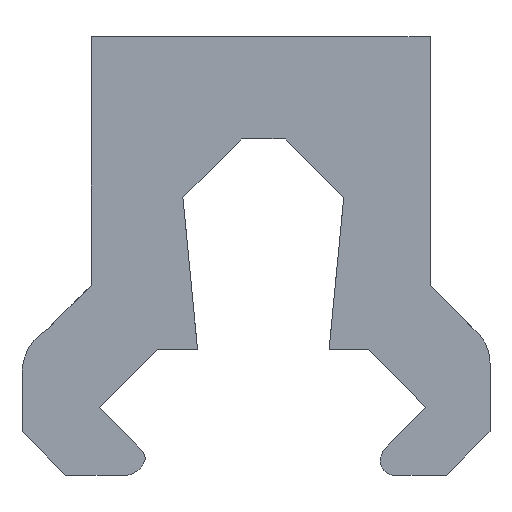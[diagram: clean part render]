
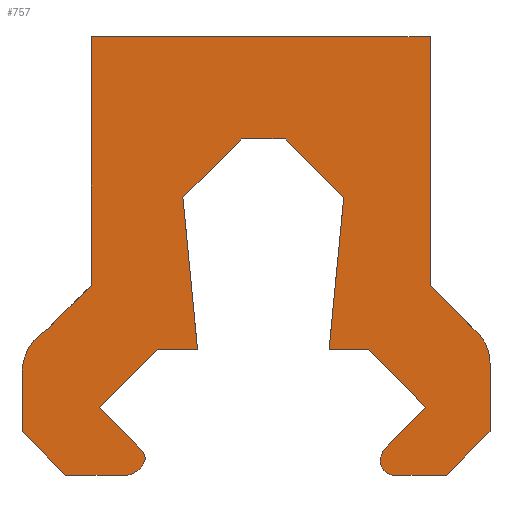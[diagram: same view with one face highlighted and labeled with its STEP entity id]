
A CAD part, left-side view. The second image highlights one B-rep face of the part: STEP entity #757.
In plain terms, the highlighted planar face has unit normal (-1, 0, 0).
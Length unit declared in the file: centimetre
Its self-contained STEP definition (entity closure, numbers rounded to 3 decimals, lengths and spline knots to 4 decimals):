
#36=LINE($,#1126,#114);
#41=LINE($,#1222,#119);
#46=LINE($,#1245,#124);
#49=LINE($,#1251,#127);
#50=LINE($,#1252,#128);
#51=LINE($,#1254,#129);
#52=LINE($,#1258,#130);
#53=LINE($,#1260,#131);
#54=LINE($,#1262,#132);
#55=LINE($,#1266,#133);
#56=LINE($,#1268,#134);
#57=LINE($,#1270,#135);
#58=LINE($,#1272,#136);
#59=LINE($,#1274,#137);
#60=LINE($,#1276,#138);
#61=LINE($,#1278,#139);
#62=LINE($,#1280,#140);
#63=LINE($,#1282,#141);
#64=LINE($,#1284,#142);
#65=LINE($,#1286,#143);
#66=LINE($,#1288,#144);
#67=LINE($,#1290,#145);
#68=LINE($,#1294,#146);
#69=LINE($,#1295,#147);
#114=VECTOR($,#853,1.7);
#119=VECTOR($,#878,0.4243);
#124=VECTOR($,#903,0.4678);
#127=VECTOR($,#908,1.7);
#128=VECTOR($,#909,2.3152);
#129=VECTOR($,#910,0.4243);
#130=VECTOR($,#913,0.397);
#131=VECTOR($,#914,0.4243);
#132=VECTOR($,#915,0.3982);
#133=VECTOR($,#918,0.0518);
#134=VECTOR($,#919,0.4193);
#135=VECTOR($,#920,0.5597);
#136=VECTOR($,#921,0.2742);
#137=VECTOR($,#922,1.0415);
#138=VECTOR($,#923,0.5657);
#139=VECTOR($,#924,0.3);
#140=VECTOR($,#925,0.5657);
#141=VECTOR($,#926,1.0415);
#142=VECTOR($,#927,0.2688);
#143=VECTOR($,#928,0.5597);
#144=VECTOR($,#929,0.4193);
#145=VECTOR($,#930,0.0346);
#146=VECTOR($,#933,0.35);
#147=VECTOR($,#934,0.4243);
#196=PLANE($,#810);
#231=CIRCLE($,#807,0.3);
#233=CIRCLE($,#811,0.35);
#234=CIRCLE($,#812,0.15);
#235=CIRCLE($,#813,0.1);
#253=FACE_OUTER_BOUND($,#297,.T.);
#297=EDGE_LOOP($,(#579,#580,#581,#582,#583,#584,#585,#586,#587,#588,#589,
#590,#591,#592,#593,#594,#595,#596,#597,#598,#599,#600,#601,#602,#603,#604,
#605,#606));
#343=VERTEX_POINT($,#1123);
#344=VERTEX_POINT($,#1125);
#356=VERTEX_POINT($,#1219);
#357=VERTEX_POINT($,#1221);
#363=VERTEX_POINT($,#1238);
#365=VERTEX_POINT($,#1244);
#367=VERTEX_POINT($,#1250);
#368=VERTEX_POINT($,#1253);
#369=VERTEX_POINT($,#1255);
#370=VERTEX_POINT($,#1257);
#371=VERTEX_POINT($,#1259);
#372=VERTEX_POINT($,#1261);
#373=VERTEX_POINT($,#1263);
#374=VERTEX_POINT($,#1265);
#375=VERTEX_POINT($,#1267);
#376=VERTEX_POINT($,#1269);
#377=VERTEX_POINT($,#1271);
#378=VERTEX_POINT($,#1273);
#379=VERTEX_POINT($,#1275);
#380=VERTEX_POINT($,#1277);
#381=VERTEX_POINT($,#1279);
#382=VERTEX_POINT($,#1281);
#383=VERTEX_POINT($,#1283);
#384=VERTEX_POINT($,#1285);
#385=VERTEX_POINT($,#1287);
#386=VERTEX_POINT($,#1289);
#387=VERTEX_POINT($,#1291);
#388=VERTEX_POINT($,#1293);
#422=EDGE_CURVE($,#344,#343,#36,.T.);
#438=EDGE_CURVE($,#357,#356,#41,.T.);
#445=EDGE_CURVE($,#357,#363,#231,.T.);
#448=EDGE_CURVE($,#363,#365,#46,.T.);
#451=EDGE_CURVE($,#356,#367,#49,.T.);
#452=EDGE_CURVE($,#344,#367,#50,.F.);
#453=EDGE_CURVE($,#343,#368,#51,.T.);
#454=EDGE_CURVE($,#369,#368,#233,.T.);
#455=EDGE_CURVE($,#370,#369,#52,.T.);
#456=EDGE_CURVE($,#371,#370,#53,.T.);
#457=EDGE_CURVE($,#372,#371,#54,.F.);
#458=EDGE_CURVE($,#373,#372,#234,.T.);
#459=EDGE_CURVE($,#374,#373,#55,.T.);
#460=EDGE_CURVE($,#375,#374,#56,.F.);
#461=EDGE_CURVE($,#376,#375,#57,.F.);
#462=EDGE_CURVE($,#377,#376,#58,.F.);
#463=EDGE_CURVE($,#377,#378,#59,.F.);
#464=EDGE_CURVE($,#379,#378,#60,.T.);
#465=EDGE_CURVE($,#379,#380,#61,.T.);
#466=EDGE_CURVE($,#381,#380,#62,.T.);
#467=EDGE_CURVE($,#381,#382,#63,.T.);
#468=EDGE_CURVE($,#383,#382,#64,.F.);
#469=EDGE_CURVE($,#384,#383,#65,.F.);
#470=EDGE_CURVE($,#385,#384,#66,.F.);
#471=EDGE_CURVE($,#386,#385,#67,.T.);
#472=EDGE_CURVE($,#387,#386,#235,.T.);
#473=EDGE_CURVE($,#388,#387,#68,.F.);
#474=EDGE_CURVE($,#365,#388,#69,.T.);
#579=ORIENTED_EDGE($,*,*,#445,.F.);
#580=ORIENTED_EDGE($,*,*,#438,.T.);
#581=ORIENTED_EDGE($,*,*,#451,.T.);
#582=ORIENTED_EDGE($,*,*,#452,.F.);
#583=ORIENTED_EDGE($,*,*,#422,.T.);
#584=ORIENTED_EDGE($,*,*,#453,.T.);
#585=ORIENTED_EDGE($,*,*,#454,.F.);
#586=ORIENTED_EDGE($,*,*,#455,.F.);
#587=ORIENTED_EDGE($,*,*,#456,.F.);
#588=ORIENTED_EDGE($,*,*,#457,.F.);
#589=ORIENTED_EDGE($,*,*,#458,.F.);
#590=ORIENTED_EDGE($,*,*,#459,.F.);
#591=ORIENTED_EDGE($,*,*,#460,.F.);
#592=ORIENTED_EDGE($,*,*,#461,.F.);
#593=ORIENTED_EDGE($,*,*,#462,.F.);
#594=ORIENTED_EDGE($,*,*,#463,.T.);
#595=ORIENTED_EDGE($,*,*,#464,.F.);
#596=ORIENTED_EDGE($,*,*,#465,.T.);
#597=ORIENTED_EDGE($,*,*,#466,.F.);
#598=ORIENTED_EDGE($,*,*,#467,.T.);
#599=ORIENTED_EDGE($,*,*,#468,.F.);
#600=ORIENTED_EDGE($,*,*,#469,.F.);
#601=ORIENTED_EDGE($,*,*,#470,.F.);
#602=ORIENTED_EDGE($,*,*,#471,.F.);
#603=ORIENTED_EDGE($,*,*,#472,.F.);
#604=ORIENTED_EDGE($,*,*,#473,.F.);
#605=ORIENTED_EDGE($,*,*,#474,.F.);
#606=ORIENTED_EDGE($,*,*,#448,.F.);
#757=ADVANCED_FACE($,(#253),#196,.F.);
#807=AXIS2_PLACEMENT_3D($,#1239,#896,#897);
#810=AXIS2_PLACEMENT_3D($,#1249,#906,#907);
#811=AXIS2_PLACEMENT_3D($,#1256,#911,#912);
#812=AXIS2_PLACEMENT_3D($,#1264,#916,#917);
#813=AXIS2_PLACEMENT_3D($,#1292,#931,#932);
#853=DIRECTION($,(0.,0.,-1.));
#878=DIRECTION($,(0.,0.707,0.707));
#896=DIRECTION('center_axis',(1.,0.,0.));
#897=DIRECTION('ref_axis',(0.,-0.633,0.774));
#903=DIRECTION($,(0.,0.,-1.));
#906=DIRECTION('center_axis',(1.,0.,0.));
#907=DIRECTION('ref_axis',(0.,0.,-1.));
#908=DIRECTION($,(0.,0.,1.));
#909=DIRECTION($,(0.,1.,0.));
#910=DIRECTION($,(0.,0.707,-0.707));
#911=DIRECTION('center_axis',(1.,0.,0.));
#912=DIRECTION('ref_axis',(0.,0.501,0.866));
#913=DIRECTION($,(0.,0.,1.));
#914=DIRECTION($,(0.,0.707,0.707));
#915=DIRECTION($,(0.,-1.,0.));
#916=DIRECTION('center_axis',(1.,0.,0.));
#917=DIRECTION('ref_axis',(0.,-0.976,-0.218));
#918=DIRECTION($,(0.,-0.335,-0.942));
#919=DIRECTION($,(0.,0.702,0.712));
#920=DIRECTION($,(0.,-0.702,0.712));
#921=DIRECTION($,(0.,-1.,0.));
#922=DIRECTION($,(0.,-0.096,-0.995));
#923=DIRECTION($,(0.,0.707,-0.707));
#924=DIRECTION($,(0.,-1.,0.));
#925=DIRECTION($,(0.,0.707,0.707));
#926=DIRECTION($,(0.,0.096,-0.995));
#927=DIRECTION($,(0.,-1.,0.));
#928=DIRECTION($,(0.,-0.702,-0.712));
#929=DIRECTION($,(0.,0.702,-0.712));
#930=DIRECTION($,(0.,-0.335,0.942));
#931=DIRECTION('center_axis',(1.,0.,0.));
#932=DIRECTION('ref_axis',(0.,0.,-1.));
#933=DIRECTION($,(0.,-1.,0.));
#934=DIRECTION($,(0.,0.707,-0.707));
#1123=CARTESIAN_POINT('',(4.,3.5252,1.9));
#1125=CARTESIAN_POINT('',(4.,3.5252,3.6));
#1126=CARTESIAN_POINT($,(4.,3.5252,2.85));
#1219=CARTESIAN_POINT('',(4.,1.21,1.9));
#1221=CARTESIAN_POINT('',(4.,0.91,1.6));
#1222=CARTESIAN_POINT($,(4.,0.8075,1.4975));
#1238=CARTESIAN_POINT('',(4.,0.8,1.3678));
#1239=CARTESIAN_POINT('Origin',(4.,1.1,1.3678));
#1244=CARTESIAN_POINT('',(4.,0.8,0.9));
#1245=CARTESIAN_POINT($,(4.,0.8,2.3));
#1249=CARTESIAN_POINT('Origin',(4.,-2.3,4.1));
#1250=CARTESIAN_POINT('',(4.,1.21,3.6));
#1251=CARTESIAN_POINT($,(4.,1.21,2.85));
#1252=CARTESIAN_POINT($,(4.,0.05,3.6));
#1253=CARTESIAN_POINT('',(4.,3.8252,1.6));
#1254=CARTESIAN_POINT($,(4.,1.5939,3.8313));
#1255=CARTESIAN_POINT('',(4.,4.,1.297));
#1256=CARTESIAN_POINT('Origin',(4.,3.65,1.297));
#1257=CARTESIAN_POINT('',(4.,4.,0.9));
#1258=CARTESIAN_POINT($,(4.,4.,2.3));
#1259=CARTESIAN_POINT('',(4.,3.7,0.6));
#1260=CARTESIAN_POINT($,(4.,3.15,0.05));
#1261=CARTESIAN_POINT('',(4.,3.3018,0.6));
#1262=CARTESIAN_POINT($,(4.,0.05,0.6));
#1263=CARTESIAN_POINT('',(4.,3.1554,0.7173));
#1264=CARTESIAN_POINT('Origin',(4.,3.3018,0.75));
#1265=CARTESIAN_POINT('',(4.,3.1727,0.7661));
#1266=CARTESIAN_POINT($,(4.,3.3651,1.3072));
#1267=CARTESIAN_POINT('',(4.,3.4671,1.0647));
#1268=CARTESIAN_POINT($,(4.,2.731,0.318));
#1269=CARTESIAN_POINT('',(4.,3.0742,1.4633));
#1270=CARTESIAN_POINT($,(4.,1.2135,3.3506));
#1271=CARTESIAN_POINT('',(4.,2.8,1.4633));
#1272=CARTESIAN_POINT($,(4.,0.0263,1.4633));
#1273=CARTESIAN_POINT('',(4.,2.9,2.5));
#1274=CARTESIAN_POINT($,(4.,2.8661,2.1483));
#1275=CARTESIAN_POINT('',(4.,2.5,2.9));
#1276=CARTESIAN_POINT($,(4.,1.1,4.3));
#1277=CARTESIAN_POINT('',(4.,2.2,2.9));
#1278=CARTESIAN_POINT($,(4.,0.3,2.9));
#1279=CARTESIAN_POINT('',(4.,1.8,2.5));
#1280=CARTESIAN_POINT($,(4.,1.275,1.975));
#1281=CARTESIAN_POINT('',(4.,1.9,1.4633));
#1282=CARTESIAN_POINT($,(4.,1.7911,2.5927));
#1283=CARTESIAN_POINT('',(4.,1.6312,1.4633));
#1284=CARTESIAN_POINT($,(4.,0.0263,1.4633));
#1285=CARTESIAN_POINT('',(4.,1.2382,1.0647));
#1286=CARTESIAN_POINT($,(4.,1.1986,1.0245));
#1287=CARTESIAN_POINT('',(4.,1.5326,0.7661));
#1288=CARTESIAN_POINT($,(4.,-0.3189,2.6441));
#1289=CARTESIAN_POINT('',(4.,1.5442,0.7335));
#1290=CARTESIAN_POINT($,(4.,0.8184,2.7755));
#1291=CARTESIAN_POINT('',(4.,1.45,0.6));
#1292=CARTESIAN_POINT('Origin',(4.,1.45,0.7));
#1293=CARTESIAN_POINT('',(4.,1.1,0.6));
#1294=CARTESIAN_POINT($,(4.,0.05,0.6));
#1295=CARTESIAN_POINT($,(4.,-0.7,2.4));
